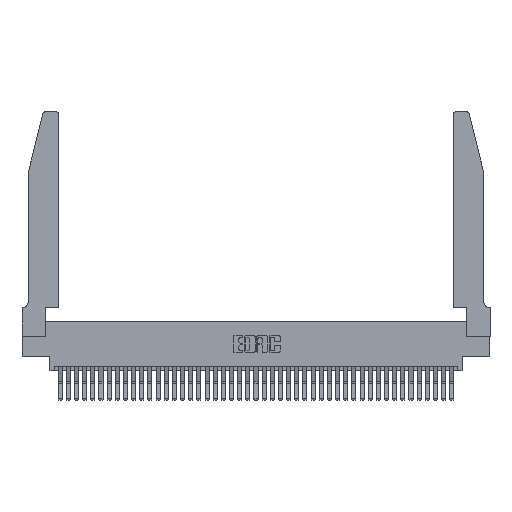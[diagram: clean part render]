
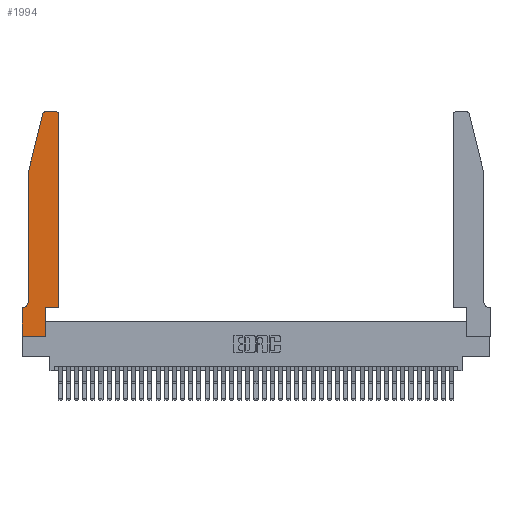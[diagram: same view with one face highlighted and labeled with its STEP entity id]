
A CAD part, top view. The second image highlights one B-rep face of the part: STEP entity #1994.
In plain terms, the highlighted planar face has unit normal (0, 0, 1).
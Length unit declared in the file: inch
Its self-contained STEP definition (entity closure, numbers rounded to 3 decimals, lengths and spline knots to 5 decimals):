
#643 = CARTESIAN_POINT ( 'NONE',  ( 0.2865, 0., 0.37 ) ) ;
#646 = CARTESIAN_POINT ( 'NONE',  ( 0.25487, 2.72718, 0.37 ) ) ;
#733 = EDGE_CURVE ( 'NONE', #12482, #16751, #36486, .T. ) ;
#1424 = VERTEX_POINT ( 'NONE', #5831 ) ;
#1540 = CARTESIAN_POINT ( 'NONE',  ( 0.4505, 0.35, 0.37 ) ) ;
#1994 = ADVANCED_FACE ( 'NONE', ( #7729 ), #37310, .T. ) ;
#2071 = DIRECTION ( 'NONE',  ( 0., 0., 1. ) ) ;
#2131 = VECTOR ( 'NONE', #30768, 39.37008 ) ;
#2408 = CIRCLE ( 'NONE', #25948, 0.07 ) ;
#2929 = VECTOR ( 'NONE', #39818, 39.37008 ) ;
#3869 = EDGE_CURVE ( 'NONE', #1424, #18897, #38298, .T. ) ;
#3951 = DIRECTION ( 'NONE',  ( 1., 0., 0. ) ) ;
#3982 = CARTESIAN_POINT ( 'NONE',  ( 0.0755, 2., 0.37 ) ) ;
#4114 = DIRECTION ( 'NONE',  ( -1., 0., 0. ) ) ;
#4170 = CARTESIAN_POINT ( 'NONE',  ( 0.0755, 2., 0.37 ) ) ;
#4507 = CIRCLE ( 'NONE', #35264, 0.03 ) ;
#5331 = DIRECTION ( 'NONE',  ( -0.239, -0.971, 0. ) ) ;
#5831 = CARTESIAN_POINT ( 'NONE',  ( 0.4205, 2.75, 0.37 ) ) ;
#6124 = ORIENTED_EDGE ( 'NONE', *, *, #14493, .T. ) ;
#6809 = DIRECTION ( 'NONE',  ( 0., 1., 0. ) ) ;
#6912 = VECTOR ( 'NONE', #24648, 39.37008 ) ;
#7041 = ORIENTED_EDGE ( 'NONE', *, *, #733, .T. ) ;
#7099 = CARTESIAN_POINT ( 'NONE',  ( 0.0055, 0.35, 0.37 ) ) ;
#7129 = VERTEX_POINT ( 'NONE', #24782 ) ;
#7399 = CARTESIAN_POINT ( 'NONE',  ( 0., 0.35, 0.37 ) ) ;
#7715 = CARTESIAN_POINT ( 'NONE',  ( 0.0055, 0.42, 0.37 ) ) ;
#7729 = FACE_OUTER_BOUND ( 'NONE', #24065, .T. ) ;
#7972 = VERTEX_POINT ( 'NONE', #37181 ) ;
#8103 = VECTOR ( 'NONE', #6809, 39.37008 ) ;
#10171 = ORIENTED_EDGE ( 'NONE', *, *, #11579, .T. ) ;
#10630 = LINE ( 'NONE', #39185, #8103 ) ;
#11579 = EDGE_CURVE ( 'NONE', #7972, #1424, #35525, .T. ) ;
#11763 = VECTOR ( 'NONE', #5331, 39.37008 ) ;
#12482 = VERTEX_POINT ( 'NONE', #16057 ) ;
#12830 = LINE ( 'NONE', #1540, #29812 ) ;
#13519 = CARTESIAN_POINT ( 'NONE',  ( 0.4505, 0.35, 0.37 ) ) ;
#13520 = LINE ( 'NONE', #34406, #6912 ) ;
#13711 = EDGE_CURVE ( 'NONE', #18897, #27700, #4507, .T. ) ;
#13901 = AXIS2_PLACEMENT_3D ( 'NONE', #7399, #30336, #3951 ) ;
#13902 = EDGE_CURVE ( 'NONE', #25491, #40536, #39371, .T. ) ;
#14224 = CARTESIAN_POINT ( 'NONE',  ( 0.0755, 0.35, 0.37 ) ) ;
#14493 = EDGE_CURVE ( 'NONE', #24029, #22177, #2408, .T. ) ;
#14702 = CARTESIAN_POINT ( 'NONE',  ( 0.4505, 0.35, 0.37 ) ) ;
#15299 = CARTESIAN_POINT ( 'NONE',  ( 0.284, 2.75, 0.37 ) ) ;
#15651 = DIRECTION ( 'NONE',  ( 1., 0., 0. ) ) ;
#16057 = CARTESIAN_POINT ( 'NONE',  ( 0.2865, 0.35, 0.37 ) ) ;
#16579 = ORIENTED_EDGE ( 'NONE', *, *, #13902, .T. ) ;
#16751 = VERTEX_POINT ( 'NONE', #13519 ) ;
#18897 = VERTEX_POINT ( 'NONE', #15299 ) ;
#19189 = AXIS2_PLACEMENT_3D ( 'NONE', #41346, #21346, #24941 ) ;
#20193 = CARTESIAN_POINT ( 'NONE',  ( 0.2605, 2.75, 0.37 ) ) ;
#20361 = ORIENTED_EDGE ( 'NONE', *, *, #30298, .T. ) ;
#21167 = CARTESIAN_POINT ( 'NONE',  ( 0.0755, 0.42, 0.37 ) ) ;
#21302 = DIRECTION ( 'NONE',  ( 0., 1., 0. ) ) ;
#21346 = DIRECTION ( 'NONE',  ( 0., 0., 1. ) ) ;
#21401 = EDGE_CURVE ( 'NONE', #27700, #37910, #34829, .T. ) ;
#21945 = CARTESIAN_POINT ( 'NONE',  ( 0., 0., 0.37 ) ) ;
#22177 = VERTEX_POINT ( 'NONE', #7099 ) ;
#22614 = EDGE_CURVE ( 'NONE', #37910, #24029, #36708, .T. ) ;
#23593 = DIRECTION ( 'NONE',  ( 0., 0., -1. ) ) ;
#23961 = EDGE_CURVE ( 'NONE', #16751, #7972, #12830, .T. ) ;
#24029 = VERTEX_POINT ( 'NONE', #21167 ) ;
#24065 = EDGE_LOOP ( 'NONE', ( #36725, #27009, #26568, #25474, #6124, #20361, #30910, #16579, #25385, #7041, #40060, #10171 ) ) ;
#24264 = VECTOR ( 'NONE', #30054, 39.37008 ) ;
#24648 = DIRECTION ( 'NONE',  ( 0., -1., 0. ) ) ;
#24782 = CARTESIAN_POINT ( 'NONE',  ( 0., 0.35, 0.37 ) ) ;
#24941 = DIRECTION ( 'NONE',  ( 1., 0., 0. ) ) ;
#24987 = CARTESIAN_POINT ( 'NONE',  ( 0.284, 2.72, 0.37 ) ) ;
#25228 = DIRECTION ( 'NONE',  ( 1., 0., 0. ) ) ;
#25385 = ORIENTED_EDGE ( 'NONE', *, *, #34071, .T. ) ;
#25474 = ORIENTED_EDGE ( 'NONE', *, *, #22614, .T. ) ;
#25491 = VERTEX_POINT ( 'NONE', #21945 ) ;
#25948 = AXIS2_PLACEMENT_3D ( 'NONE', #7715, #23593, #4114 ) ;
#26353 = LINE ( 'NONE', #14224, #24264 ) ;
#26568 = ORIENTED_EDGE ( 'NONE', *, *, #21401, .T. ) ;
#27009 = ORIENTED_EDGE ( 'NONE', *, *, #13711, .T. ) ;
#27519 = VECTOR ( 'NONE', #39267, 39.37008 ) ;
#27700 = VERTEX_POINT ( 'NONE', #646 ) ;
#29812 = VECTOR ( 'NONE', #21302, 39.37008 ) ;
#30054 = DIRECTION ( 'NONE',  ( -1., 0., 0. ) ) ;
#30298 = EDGE_CURVE ( 'NONE', #22177, #7129, #26353, .T. ) ;
#30336 = DIRECTION ( 'NONE',  ( 0., 0., 1. ) ) ;
#30768 = DIRECTION ( 'NONE',  ( 1., 0., 0. ) ) ;
#30910 = ORIENTED_EDGE ( 'NONE', *, *, #41906, .T. ) ;
#34071 = EDGE_CURVE ( 'NONE', #40536, #12482, #10630, .T. ) ;
#34259 = VECTOR ( 'NONE', #25228, 39.37008 ) ;
#34406 = CARTESIAN_POINT ( 'NONE',  ( 0., 0., 0.37 ) ) ;
#34829 = LINE ( 'NONE', #4170, #11763 ) ;
#34979 = CARTESIAN_POINT ( 'NONE',  ( 0., 0., 0.37 ) ) ;
#35264 = AXIS2_PLACEMENT_3D ( 'NONE', #24987, #2071, #15651 ) ;
#35525 = CIRCLE ( 'NONE', #19189, 0.03 ) ;
#36486 = LINE ( 'NONE', #14702, #2131 ) ;
#36708 = LINE ( 'NONE', #41249, #27519 ) ;
#36725 = ORIENTED_EDGE ( 'NONE', *, *, #3869, .T. ) ;
#37181 = CARTESIAN_POINT ( 'NONE',  ( 0.4505, 2.72, 0.37 ) ) ;
#37310 = PLANE ( 'NONE',  #13901 ) ;
#37910 = VERTEX_POINT ( 'NONE', #3982 ) ;
#38298 = LINE ( 'NONE', #20193, #2929 ) ;
#39185 = CARTESIAN_POINT ( 'NONE',  ( 0.2865, 0.35, 0.37 ) ) ;
#39267 = DIRECTION ( 'NONE',  ( 0., -1., 0. ) ) ;
#39371 = LINE ( 'NONE', #34979, #34259 ) ;
#39818 = DIRECTION ( 'NONE',  ( -1., 0., 0. ) ) ;
#40060 = ORIENTED_EDGE ( 'NONE', *, *, #23961, .T. ) ;
#40536 = VERTEX_POINT ( 'NONE', #643 ) ;
#41249 = CARTESIAN_POINT ( 'NONE',  ( 0.0755, 2., 0.37 ) ) ;
#41346 = CARTESIAN_POINT ( 'NONE',  ( 0.4205, 2.72, 0.37 ) ) ;
#41906 = EDGE_CURVE ( 'NONE', #7129, #25491, #13520, .T. ) ;
